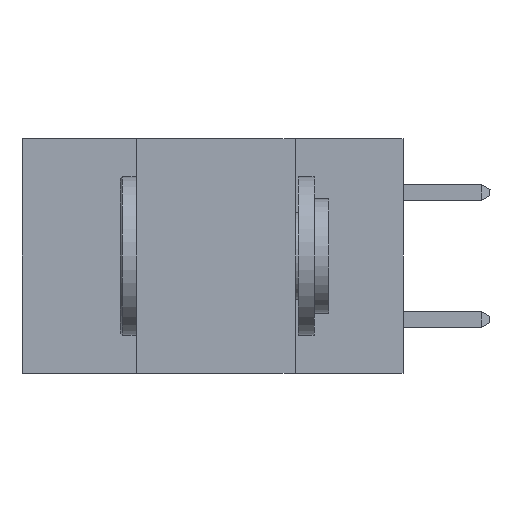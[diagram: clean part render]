
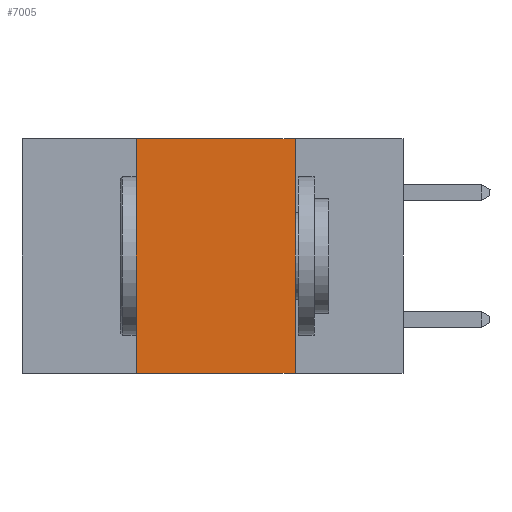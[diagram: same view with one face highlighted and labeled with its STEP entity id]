
A CAD part, left-side view. The second image highlights one B-rep face of the part: STEP entity #7005.
In plain terms, the highlighted planar face has unit normal (-1, 0, 0).
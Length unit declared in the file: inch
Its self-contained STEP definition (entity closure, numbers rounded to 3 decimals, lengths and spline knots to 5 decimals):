
#730 = EDGE_CURVE ( 'NONE', #8161, #13252, #6119, .T. ) ;
#1070 = VERTEX_POINT ( 'NONE', #10801 ) ;
#1563 = ORIENTED_EDGE ( 'NONE', *, *, #730, .F. ) ;
#1877 = CARTESIAN_POINT ( 'NONE',  ( 0., 0.6, 0. ) ) ;
#1881 = AXIS2_PLACEMENT_3D ( 'NONE', #1877, #12894, #4930 ) ;
#2523 = VECTOR ( 'NONE', #2752, 39.37008 ) ;
#2581 = ORIENTED_EDGE ( 'NONE', *, *, #14619, .F. ) ;
#2752 = DIRECTION ( 'NONE',  ( 0., -1., 0. ) ) ;
#3038 = EDGE_CURVE ( 'NONE', #8161, #8512, #3115, .T. ) ;
#3115 = LINE ( 'NONE', #12981, #17065 ) ;
#3349 = CARTESIAN_POINT ( 'NONE',  ( 0., 0.17, 0. ) ) ;
#3747 = DIRECTION ( 'NONE',  ( 0., 0., -1. ) ) ;
#4236 = FACE_OUTER_BOUND ( 'NONE', #11846, .T. ) ;
#4930 = DIRECTION ( 'NONE',  ( 0., 0., -1. ) ) ;
#5204 = LINE ( 'NONE', #3349, #16378 ) ;
#5230 = VECTOR ( 'NONE', #15125, 39.37008 ) ;
#6119 = LINE ( 'NONE', #15010, #5230 ) ;
#6188 = LINE ( 'NONE', #9627, #2523 ) ;
#7005 = ADVANCED_FACE ( 'NONE', ( #4236 ), #11438, .F. ) ;
#8161 = VERTEX_POINT ( 'NONE', #8458 ) ;
#8458 = CARTESIAN_POINT ( 'NONE',  ( 0., 0.42, -0.37 ) ) ;
#8512 = VERTEX_POINT ( 'NONE', #14376 ) ;
#9627 = CARTESIAN_POINT ( 'NONE',  ( 0., 0.6, 0. ) ) ;
#10801 = CARTESIAN_POINT ( 'NONE',  ( 0., 0.17, 0. ) ) ;
#10883 = CARTESIAN_POINT ( 'NONE',  ( 0., 0.42, 0. ) ) ;
#11438 = PLANE ( 'NONE',  #1881 ) ;
#11846 = EDGE_LOOP ( 'NONE', ( #16626, #2581, #1563, #13699 ) ) ;
#12894 = DIRECTION ( 'NONE',  ( 1., 0., 0. ) ) ;
#12981 = CARTESIAN_POINT ( 'NONE',  ( 0., 0.6, -0.37 ) ) ;
#13252 = VERTEX_POINT ( 'NONE', #10883 ) ;
#13699 = ORIENTED_EDGE ( 'NONE', *, *, #3038, .T. ) ;
#14376 = CARTESIAN_POINT ( 'NONE',  ( 0., 0.17, -0.37 ) ) ;
#14616 = DIRECTION ( 'NONE',  ( 0., -1., 0. ) ) ;
#14619 = EDGE_CURVE ( 'NONE', #13252, #1070, #6188, .T. ) ;
#15010 = CARTESIAN_POINT ( 'NONE',  ( 0., 0.42, 0. ) ) ;
#15125 = DIRECTION ( 'NONE',  ( 0., 0., 1. ) ) ;
#16378 = VECTOR ( 'NONE', #3747, 39.37008 ) ;
#16626 = ORIENTED_EDGE ( 'NONE', *, *, #17093, .F. ) ;
#17065 = VECTOR ( 'NONE', #14616, 39.37008 ) ;
#17093 = EDGE_CURVE ( 'NONE', #1070, #8512, #5204, .T. ) ;
